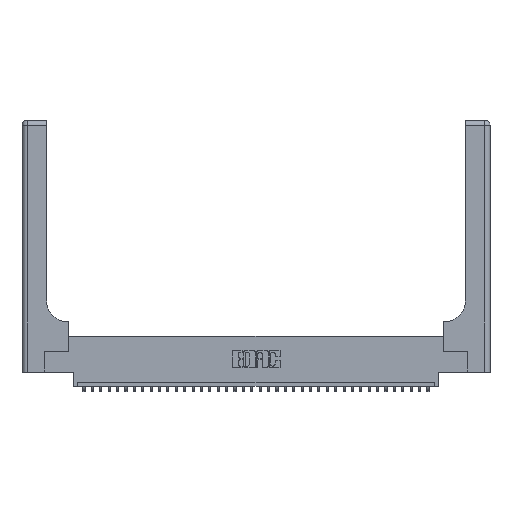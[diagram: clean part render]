
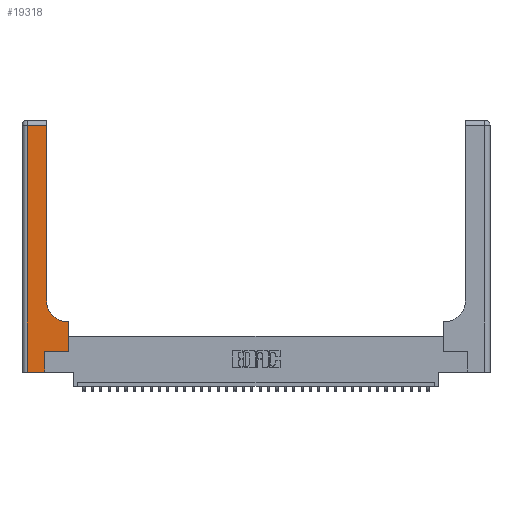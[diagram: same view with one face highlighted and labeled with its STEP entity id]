
A CAD part, top view. The second image highlights one B-rep face of the part: STEP entity #19318.
In plain terms, the highlighted planar face has unit normal (0, 0, 1).
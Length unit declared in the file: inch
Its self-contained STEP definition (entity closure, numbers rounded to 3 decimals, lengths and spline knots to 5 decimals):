
#227 = CARTESIAN_POINT ( 'NONE',  ( 0.269, 0.25, 0.37 ) ) ;
#1134 = CARTESIAN_POINT ( 'NONE',  ( 0.2915, 0.6, 0.37 ) ) ;
#1467 = CARTESIAN_POINT ( 'NONE',  ( 0.5585, 0.25, 0.37 ) ) ;
#1731 = CARTESIAN_POINT ( 'NONE',  ( 0., 2.94, 0.37 ) ) ;
#1918 = CARTESIAN_POINT ( 'NONE',  ( 0.2915, 3., 0.37 ) ) ;
#2779 = VECTOR ( 'NONE', #21974, 39.37008 ) ;
#2889 = EDGE_CURVE ( 'NONE', #5769, #13606, #25628, .T. ) ;
#3456 = VERTEX_POINT ( 'NONE', #33679 ) ;
#3623 = CARTESIAN_POINT ( 'NONE',  ( 0.2915, 2.94, 0.37 ) ) ;
#3958 = VERTEX_POINT ( 'NONE', #7117 ) ;
#4077 = DIRECTION ( 'NONE',  ( 0., 1., 0. ) ) ;
#5769 = VERTEX_POINT ( 'NONE', #28624 ) ;
#5926 = ORIENTED_EDGE ( 'NONE', *, *, #7937, .T. ) ;
#6092 = VERTEX_POINT ( 'NONE', #1467 ) ;
#6176 = EDGE_CURVE ( 'NONE', #13606, #24268, #32554, .T. ) ;
#6276 = DIRECTION ( 'NONE',  ( 0., 0., -1. ) ) ;
#6419 = VECTOR ( 'NONE', #32800, 39.37008 ) ;
#7117 = CARTESIAN_POINT ( 'NONE',  ( 0.5585, 0.6, 0.37 ) ) ;
#7144 = EDGE_CURVE ( 'NONE', #3456, #34748, #23988, .T. ) ;
#7210 = ORIENTED_EDGE ( 'NONE', *, *, #7144, .T. ) ;
#7298 = LINE ( 'NONE', #29027, #22564 ) ;
#7937 = EDGE_CURVE ( 'NONE', #3958, #15616, #35074, .T. ) ;
#8532 = AXIS2_PLACEMENT_3D ( 'NONE', #14403, #31689, #9114 ) ;
#8734 = EDGE_CURVE ( 'NONE', #6092, #3958, #10346, .T. ) ;
#8907 = ORIENTED_EDGE ( 'NONE', *, *, #36447, .T. ) ;
#9114 = DIRECTION ( 'NONE',  ( -1., 0., 0. ) ) ;
#9463 = FACE_OUTER_BOUND ( 'NONE', #32077, .T. ) ;
#9630 = CARTESIAN_POINT ( 'NONE',  ( 0.269, 0.25, 0.37 ) ) ;
#10346 = LINE ( 'NONE', #12061, #20645 ) ;
#11670 = VERTEX_POINT ( 'NONE', #9630 ) ;
#12061 = CARTESIAN_POINT ( 'NONE',  ( 0.5585, 0.25, 0.37 ) ) ;
#13606 = VERTEX_POINT ( 'NONE', #3623 ) ;
#14342 = ORIENTED_EDGE ( 'NONE', *, *, #2889, .T. ) ;
#14403 = CARTESIAN_POINT ( 'NONE',  ( 0., 3., 0.37 ) ) ;
#14595 = CARTESIAN_POINT ( 'NONE',  ( 0.5415, 0.6, 0.37 ) ) ;
#14950 = VECTOR ( 'NONE', #22914, 39.37008 ) ;
#15616 = VERTEX_POINT ( 'NONE', #14595 ) ;
#16139 = DIRECTION ( 'NONE',  ( 0., -1., 0. ) ) ;
#16421 = VECTOR ( 'NONE', #21776, 39.37008 ) ;
#16611 = VECTOR ( 'NONE', #16139, 39.37008 ) ;
#17047 = LINE ( 'NONE', #227, #34492 ) ;
#19318 = ADVANCED_FACE ( 'NONE', ( #9463 ), #23176, .F. ) ;
#19619 = EDGE_CURVE ( 'NONE', #24268, #3456, #26948, .T. ) ;
#19946 = EDGE_CURVE ( 'NONE', #11670, #6092, #17047, .T. ) ;
#20245 = DIRECTION ( 'NONE',  ( 1., 0., 0. ) ) ;
#20645 = VECTOR ( 'NONE', #4077, 39.37008 ) ;
#20848 = CARTESIAN_POINT ( 'NONE',  ( 0.06, 2.94, 0.37 ) ) ;
#21776 = DIRECTION ( 'NONE',  ( -1., 0., 0. ) ) ;
#21974 = DIRECTION ( 'NONE',  ( 0., 1., 0. ) ) ;
#22564 = VECTOR ( 'NONE', #34998, 39.37008 ) ;
#22783 = CARTESIAN_POINT ( 'NONE',  ( 0.269, 0., 0.37 ) ) ;
#22914 = DIRECTION ( 'NONE',  ( 1., 0., 0. ) ) ;
#23176 = PLANE ( 'NONE',  #8532 ) ;
#23440 = CARTESIAN_POINT ( 'NONE',  ( 0.5415, 0.85, 0.37 ) ) ;
#23988 = LINE ( 'NONE', #35746, #14950 ) ;
#24268 = VERTEX_POINT ( 'NONE', #20848 ) ;
#24540 = CARTESIAN_POINT ( 'NONE',  ( 0.06, 3., 0.37 ) ) ;
#24894 = AXIS2_PLACEMENT_3D ( 'NONE', #23440, #6276, #26190 ) ;
#25429 = ORIENTED_EDGE ( 'NONE', *, *, #19619, .T. ) ;
#25628 = LINE ( 'NONE', #1918, #2779 ) ;
#26190 = DIRECTION ( 'NONE',  ( 1., 0., 0. ) ) ;
#26948 = LINE ( 'NONE', #24540, #16611 ) ;
#28206 = ORIENTED_EDGE ( 'NONE', *, *, #19946, .T. ) ;
#28624 = CARTESIAN_POINT ( 'NONE',  ( 0.2915, 0.85, 0.37 ) ) ;
#28801 = CIRCLE ( 'NONE', #24894, 0.25 ) ;
#29027 = CARTESIAN_POINT ( 'NONE',  ( 0.269, 0., 0.37 ) ) ;
#31689 = DIRECTION ( 'NONE',  ( 0., 0., -1. ) ) ;
#32077 = EDGE_LOOP ( 'NONE', ( #14342, #33634, #25429, #7210, #32141, #28206, #36301, #5926, #8907 ) ) ;
#32141 = ORIENTED_EDGE ( 'NONE', *, *, #36032, .T. ) ;
#32554 = LINE ( 'NONE', #1731, #16421 ) ;
#32800 = DIRECTION ( 'NONE',  ( -1., 0., 0. ) ) ;
#33634 = ORIENTED_EDGE ( 'NONE', *, *, #6176, .T. ) ;
#33679 = CARTESIAN_POINT ( 'NONE',  ( 0.06, 0., 0.37 ) ) ;
#34492 = VECTOR ( 'NONE', #20245, 39.37008 ) ;
#34748 = VERTEX_POINT ( 'NONE', #22783 ) ;
#34998 = DIRECTION ( 'NONE',  ( 0., 1., 0. ) ) ;
#35074 = LINE ( 'NONE', #1134, #6419 ) ;
#35746 = CARTESIAN_POINT ( 'NONE',  ( 0., 0., 0.37 ) ) ;
#36032 = EDGE_CURVE ( 'NONE', #34748, #11670, #7298, .T. ) ;
#36301 = ORIENTED_EDGE ( 'NONE', *, *, #8734, .T. ) ;
#36447 = EDGE_CURVE ( 'NONE', #15616, #5769, #28801, .T. ) ;
